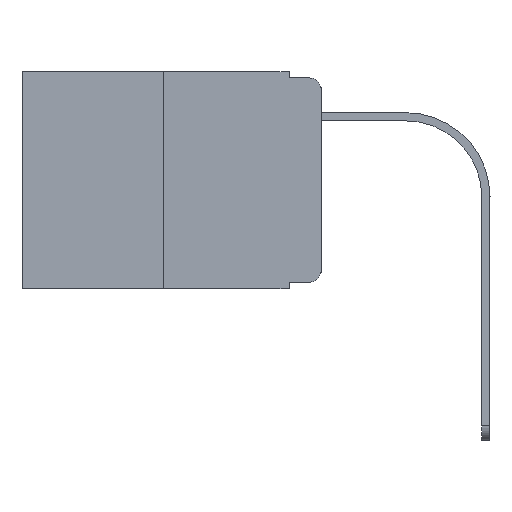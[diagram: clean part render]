
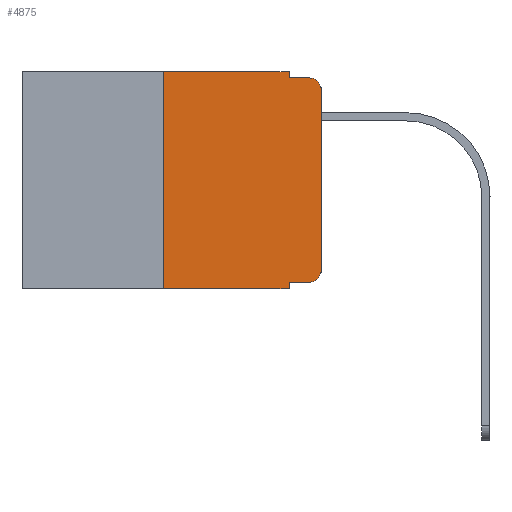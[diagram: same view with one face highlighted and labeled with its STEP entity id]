
A CAD part, left-side view. The second image highlights one B-rep face of the part: STEP entity #4875.
In plain terms, the highlighted planar face has unit normal (-1, 0, 0).
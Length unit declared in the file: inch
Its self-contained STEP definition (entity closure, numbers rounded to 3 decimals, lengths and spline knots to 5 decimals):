
#377 = LINE ( 'NONE', #7014, #9301 ) ;
#476 = DIRECTION ( 'NONE',  ( 0., -1., 0. ) ) ;
#524 = ORIENTED_EDGE ( 'NONE', *, *, #8023, .T. ) ;
#530 = DIRECTION ( 'NONE',  ( 1., 0., 0. ) ) ;
#643 = EDGE_CURVE ( 'NONE', #8067, #5882, #11467, .T. ) ;
#683 = CARTESIAN_POINT ( 'NONE',  ( 0., 0., -0.03 ) ) ;
#766 = VERTEX_POINT ( 'NONE', #5692 ) ;
#931 = VERTEX_POINT ( 'NONE', #4982 ) ;
#1149 = ORIENTED_EDGE ( 'NONE', *, *, #8573, .T. ) ;
#1406 = CARTESIAN_POINT ( 'NONE',  ( 0., 0.051, -0.333 ) ) ;
#1429 = EDGE_CURVE ( 'NONE', #5384, #766, #4682, .T. ) ;
#1645 = VECTOR ( 'NONE', #7886, 39.37008 ) ;
#1657 = CARTESIAN_POINT ( 'NONE',  ( 0., 0.051, 0. ) ) ;
#1675 = EDGE_CURVE ( 'NONE', #4031, #7207, #10010, .T. ) ;
#1715 = DIRECTION ( 'NONE',  ( 0., 0., -1. ) ) ;
#1802 = VERTEX_POINT ( 'NONE', #12300 ) ;
#2053 = DIRECTION ( 'NONE',  ( 0., -1., 0. ) ) ;
#2478 = ORIENTED_EDGE ( 'NONE', *, *, #1675, .F. ) ;
#2651 = CARTESIAN_POINT ( 'NONE',  ( 0., 0.051, 0. ) ) ;
#2689 = CARTESIAN_POINT ( 'NONE',  ( 0., 0.051, -0.01 ) ) ;
#2694 = DIRECTION ( 'NONE',  ( 0., -1., 0. ) ) ;
#3043 = VECTOR ( 'NONE', #476, 39.37008 ) ;
#3186 = EDGE_CURVE ( 'NONE', #931, #7113, #6724, .T. ) ;
#3801 = CARTESIAN_POINT ( 'NONE',  ( 0., 0.02, -0.313 ) ) ;
#3983 = CIRCLE ( 'NONE', #10971, 0.02 ) ;
#4009 = ORIENTED_EDGE ( 'NONE', *, *, #3186, .T. ) ;
#4031 = VERTEX_POINT ( 'NONE', #10793 ) ;
#4120 = EDGE_LOOP ( 'NONE', ( #4009, #10818, #6400, #6682, #10015, #2478, #1149, #11657, #524, #11718 ) ) ;
#4682 = LINE ( 'NONE', #2651, #6238 ) ;
#4862 = CARTESIAN_POINT ( 'NONE',  ( 0., 0.02, -0.01 ) ) ;
#4875 = ADVANCED_FACE ( 'NONE', ( #12290 ), #5359, .F. ) ;
#4982 = CARTESIAN_POINT ( 'NONE',  ( 0., 0., -0.313 ) ) ;
#5012 = LINE ( 'NONE', #6995, #6847 ) ;
#5359 = PLANE ( 'NONE',  #7323 ) ;
#5384 = VERTEX_POINT ( 'NONE', #1406 ) ;
#5692 = CARTESIAN_POINT ( 'NONE',  ( 0., 0.051, -0.343 ) ) ;
#5882 = VERTEX_POINT ( 'NONE', #4862 ) ;
#6128 = EDGE_CURVE ( 'NONE', #7113, #5882, #6484, .T. ) ;
#6238 = VECTOR ( 'NONE', #12315, 39.37008 ) ;
#6251 = EDGE_CURVE ( 'NONE', #7207, #1802, #9598, .T. ) ;
#6400 = ORIENTED_EDGE ( 'NONE', *, *, #643, .F. ) ;
#6429 = VERTEX_POINT ( 'NONE', #11000 ) ;
#6455 = DIRECTION ( 'NONE',  ( 0., 0., -1. ) ) ;
#6484 = CIRCLE ( 'NONE', #10370, 0.02 ) ;
#6682 = ORIENTED_EDGE ( 'NONE', *, *, #11960, .F. ) ;
#6724 = LINE ( 'NONE', #12623, #1645 ) ;
#6756 = DIRECTION ( 'NONE',  ( -1., 0., 0. ) ) ;
#6847 = VECTOR ( 'NONE', #2694, 39.37008 ) ;
#6995 = CARTESIAN_POINT ( 'NONE',  ( 0., 0.473, -0.343 ) ) ;
#7014 = CARTESIAN_POINT ( 'NONE',  ( 0., 0.051, -0.333 ) ) ;
#7113 = VERTEX_POINT ( 'NONE', #683 ) ;
#7207 = VERTEX_POINT ( 'NONE', #9824 ) ;
#7297 = DIRECTION ( 'NONE',  ( 0., 0., -1. ) ) ;
#7323 = AXIS2_PLACEMENT_3D ( 'NONE', #7361, #530, #7297 ) ;
#7361 = CARTESIAN_POINT ( 'NONE',  ( 0., 0.473, 0. ) ) ;
#7414 = VECTOR ( 'NONE', #2053, 39.37008 ) ;
#7886 = DIRECTION ( 'NONE',  ( 0., 0., 1. ) ) ;
#8023 = EDGE_CURVE ( 'NONE', #5384, #6429, #377, .T. ) ;
#8067 = VERTEX_POINT ( 'NONE', #10863 ) ;
#8213 = CARTESIAN_POINT ( 'NONE',  ( 0., 0.25, 0. ) ) ;
#8447 = DIRECTION ( 'NONE',  ( -1., 0., 0. ) ) ;
#8573 = EDGE_CURVE ( 'NONE', #4031, #766, #5012, .T. ) ;
#9109 = EDGE_CURVE ( 'NONE', #6429, #931, #3983, .T. ) ;
#9228 = DIRECTION ( 'NONE',  ( 0., 0., 1. ) ) ;
#9278 = CARTESIAN_POINT ( 'NONE',  ( 0., 0.02, -0.03 ) ) ;
#9301 = VECTOR ( 'NONE', #11120, 39.37008 ) ;
#9598 = LINE ( 'NONE', #11584, #7414 ) ;
#9824 = CARTESIAN_POINT ( 'NONE',  ( 0., 0.25, 0. ) ) ;
#10010 = LINE ( 'NONE', #8213, #11165 ) ;
#10015 = ORIENTED_EDGE ( 'NONE', *, *, #6251, .F. ) ;
#10370 = AXIS2_PLACEMENT_3D ( 'NONE', #9278, #8447, #6455 ) ;
#10664 = DIRECTION ( 'NONE',  ( 0., 0., -1. ) ) ;
#10793 = CARTESIAN_POINT ( 'NONE',  ( 0., 0.25, -0.343 ) ) ;
#10818 = ORIENTED_EDGE ( 'NONE', *, *, #6128, .T. ) ;
#10863 = CARTESIAN_POINT ( 'NONE',  ( 0., 0.051, -0.01 ) ) ;
#10971 = AXIS2_PLACEMENT_3D ( 'NONE', #3801, #6756, #10664 ) ;
#11000 = CARTESIAN_POINT ( 'NONE',  ( 0., 0.02, -0.333 ) ) ;
#11120 = DIRECTION ( 'NONE',  ( 0., -1., 0. ) ) ;
#11165 = VECTOR ( 'NONE', #9228, 39.37008 ) ;
#11467 = LINE ( 'NONE', #2689, #3043 ) ;
#11496 = VECTOR ( 'NONE', #1715, 39.37008 ) ;
#11584 = CARTESIAN_POINT ( 'NONE',  ( 0., 0.473, 0. ) ) ;
#11657 = ORIENTED_EDGE ( 'NONE', *, *, #1429, .F. ) ;
#11718 = ORIENTED_EDGE ( 'NONE', *, *, #9109, .T. ) ;
#11960 = EDGE_CURVE ( 'NONE', #1802, #8067, #12345, .T. ) ;
#12290 = FACE_OUTER_BOUND ( 'NONE', #4120, .T. ) ;
#12300 = CARTESIAN_POINT ( 'NONE',  ( 0., 0.051, 0. ) ) ;
#12315 = DIRECTION ( 'NONE',  ( 0., 0., -1. ) ) ;
#12345 = LINE ( 'NONE', #1657, #11496 ) ;
#12623 = CARTESIAN_POINT ( 'NONE',  ( 0., 0., 0. ) ) ;
